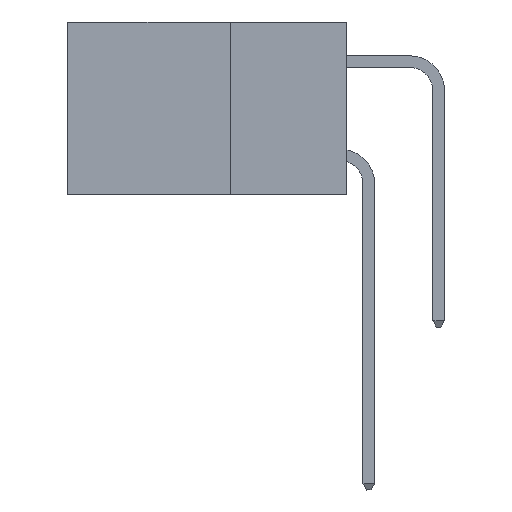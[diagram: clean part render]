
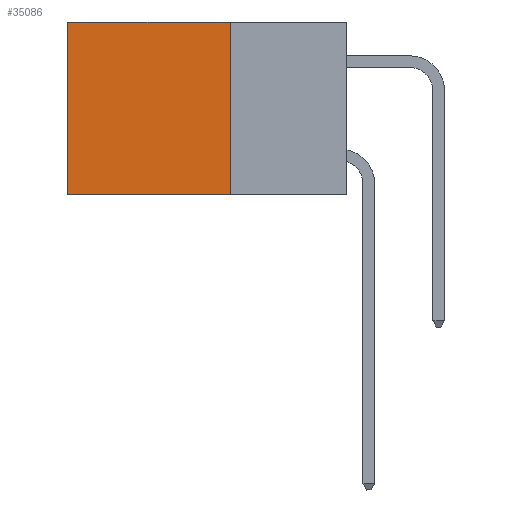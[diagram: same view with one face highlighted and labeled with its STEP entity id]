
A CAD part, left-side view. The second image highlights one B-rep face of the part: STEP entity #35086.
In plain terms, the highlighted planar face has unit normal (-1, 0, 0).
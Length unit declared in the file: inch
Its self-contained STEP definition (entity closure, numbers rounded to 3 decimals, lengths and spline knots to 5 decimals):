
#663 = VERTEX_POINT ( 'NONE', #15007 ) ;
#1675 = DIRECTION ( 'NONE',  ( 0., 0., -1. ) ) ;
#3368 = LINE ( 'NONE', #11968, #16260 ) ;
#3861 = EDGE_CURVE ( 'NONE', #31133, #16102, #20857, .T. ) ;
#5769 = VECTOR ( 'NONE', #1675, 39.37008 ) ;
#6911 = CARTESIAN_POINT ( 'NONE',  ( 0.2875, 0.6, 0. ) ) ;
#7709 = FACE_OUTER_BOUND ( 'NONE', #21035, .T. ) ;
#11968 = CARTESIAN_POINT ( 'NONE',  ( 0.2875, 0.25, -0.37 ) ) ;
#12512 = LINE ( 'NONE', #37077, #28030 ) ;
#15007 = CARTESIAN_POINT ( 'NONE',  ( 0.2875, 0.6, 0. ) ) ;
#15422 = LINE ( 'NONE', #6911, #5769 ) ;
#16102 = VERTEX_POINT ( 'NONE', #20066 ) ;
#16260 = VECTOR ( 'NONE', #29059, 39.37008 ) ;
#16565 = ORIENTED_EDGE ( 'NONE', *, *, #28982, .T. ) ;
#17179 = ORIENTED_EDGE ( 'NONE', *, *, #37259, .F. ) ;
#17472 = VERTEX_POINT ( 'NONE', #19039 ) ;
#19039 = CARTESIAN_POINT ( 'NONE',  ( 0.2875, 0.6, -0.37 ) ) ;
#20066 = CARTESIAN_POINT ( 'NONE',  ( 0.2875, 0.25, -0.37 ) ) ;
#20619 = ORIENTED_EDGE ( 'NONE', *, *, #20718, .T. ) ;
#20718 = EDGE_CURVE ( 'NONE', #31133, #663, #12512, .T. ) ;
#20857 = LINE ( 'NONE', #35905, #37254 ) ;
#21035 = EDGE_LOOP ( 'NONE', ( #16565, #17179, #23384, #20619 ) ) ;
#22925 = CARTESIAN_POINT ( 'NONE',  ( 0.2875, 0.25, 0. ) ) ;
#23384 = ORIENTED_EDGE ( 'NONE', *, *, #3861, .F. ) ;
#25840 = DIRECTION ( 'NONE',  ( 1., 0., 0. ) ) ;
#28030 = VECTOR ( 'NONE', #28438, 39.37008 ) ;
#28438 = DIRECTION ( 'NONE',  ( 0., 1., 0. ) ) ;
#28542 = PLANE ( 'NONE',  #34714 ) ;
#28982 = EDGE_CURVE ( 'NONE', #663, #17472, #15422, .T. ) ;
#29059 = DIRECTION ( 'NONE',  ( 0., 1., 0. ) ) ;
#30743 = DIRECTION ( 'NONE',  ( 0., 0., -1. ) ) ;
#31133 = VERTEX_POINT ( 'NONE', #33816 ) ;
#31686 = DIRECTION ( 'NONE',  ( 0., 0., -1. ) ) ;
#33816 = CARTESIAN_POINT ( 'NONE',  ( 0.2875, 0.25, 0. ) ) ;
#34714 = AXIS2_PLACEMENT_3D ( 'NONE', #22925, #25840, #31686 ) ;
#35086 = ADVANCED_FACE ( 'NONE', ( #7709 ), #28542, .F. ) ;
#35905 = CARTESIAN_POINT ( 'NONE',  ( 0.2875, 0.25, 0. ) ) ;
#37077 = CARTESIAN_POINT ( 'NONE',  ( 0.2875, 0.25, 0. ) ) ;
#37254 = VECTOR ( 'NONE', #30743, 39.37008 ) ;
#37259 = EDGE_CURVE ( 'NONE', #16102, #17472, #3368, .T. ) ;
